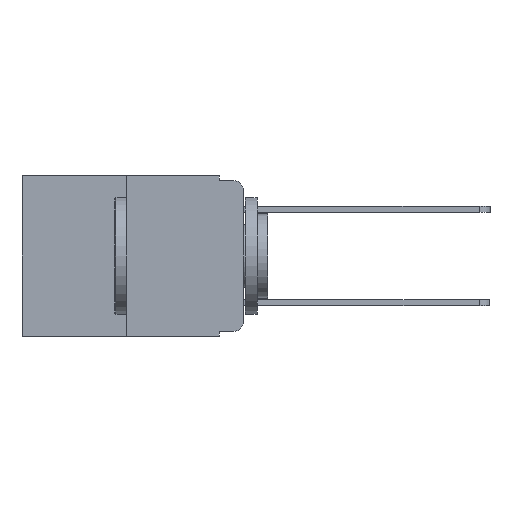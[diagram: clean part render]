
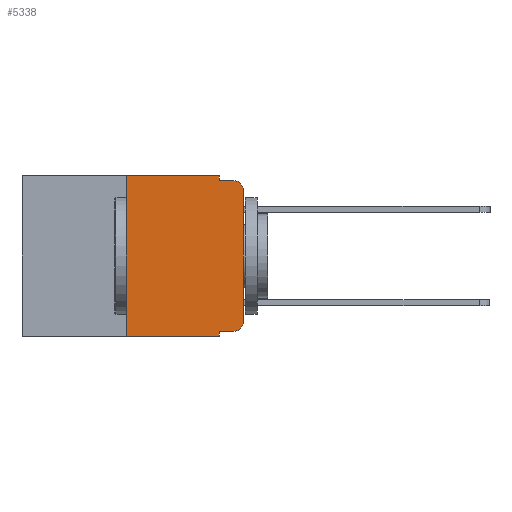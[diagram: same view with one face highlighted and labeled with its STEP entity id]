
A CAD part, left-side view. The second image highlights one B-rep face of the part: STEP entity #5338.
In plain terms, the highlighted planar face has unit normal (-1, 0, 0).
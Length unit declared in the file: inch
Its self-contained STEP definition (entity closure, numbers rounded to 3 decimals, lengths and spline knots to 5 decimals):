
#189 = CIRCLE ( 'NONE', #2507, 0.02 ) ;
#321 = EDGE_CURVE ( 'NONE', #970, #2202, #3311, .T. ) ;
#327 = ORIENTED_EDGE ( 'NONE', *, *, #11751, .T. ) ;
#368 = CARTESIAN_POINT ( 'NONE',  ( 0., 0.473, 0. ) ) ;
#484 = VERTEX_POINT ( 'NONE', #5245 ) ;
#970 = VERTEX_POINT ( 'NONE', #9499 ) ;
#1048 = EDGE_CURVE ( 'NONE', #1495, #7305, #7095, .T. ) ;
#1229 = EDGE_CURVE ( 'NONE', #1495, #2202, #2308, .T. ) ;
#1413 = CARTESIAN_POINT ( 'NONE',  ( 0., 0.02, -0.03 ) ) ;
#1495 = VERTEX_POINT ( 'NONE', #3826 ) ;
#1703 = AXIS2_PLACEMENT_3D ( 'NONE', #368, #11170, #5492 ) ;
#1918 = CARTESIAN_POINT ( 'NONE',  ( 0., 0.051, -0.01 ) ) ;
#1962 = VERTEX_POINT ( 'NONE', #1918 ) ;
#2202 = VERTEX_POINT ( 'NONE', #9196 ) ;
#2308 = LINE ( 'NONE', #10775, #7242 ) ;
#2401 = CARTESIAN_POINT ( 'NONE',  ( 0., 0.02, -0.01 ) ) ;
#2425 = FACE_OUTER_BOUND ( 'NONE', #11619, .T. ) ;
#2480 = EDGE_CURVE ( 'NONE', #5399, #1962, #8174, .T. ) ;
#2504 = DIRECTION ( 'NONE',  ( 0., 0., -1. ) ) ;
#2507 = AXIS2_PLACEMENT_3D ( 'NONE', #4015, #10698, #4992 ) ;
#2570 = PLANE ( 'NONE',  #1703 ) ;
#2672 = CARTESIAN_POINT ( 'NONE',  ( 0., 0., 0. ) ) ;
#3140 = VECTOR ( 'NONE', #8486, 39.37008 ) ;
#3311 = LINE ( 'NONE', #6581, #3622 ) ;
#3426 = CARTESIAN_POINT ( 'NONE',  ( 0., 0.051, 0. ) ) ;
#3622 = VECTOR ( 'NONE', #11095, 39.37008 ) ;
#3826 = CARTESIAN_POINT ( 'NONE',  ( 0., 0.25, -0.343 ) ) ;
#4003 = DIRECTION ( 'NONE',  ( 0., -1., 0. ) ) ;
#4015 = CARTESIAN_POINT ( 'NONE',  ( 0., 0.02, -0.313 ) ) ;
#4324 = DIRECTION ( 'NONE',  ( 0., -1., 0. ) ) ;
#4512 = EDGE_CURVE ( 'NONE', #1962, #9073, #8993, .T. ) ;
#4585 = ORIENTED_EDGE ( 'NONE', *, *, #6450, .T. ) ;
#4618 = CARTESIAN_POINT ( 'NONE',  ( 0., 0.25, 0. ) ) ;
#4736 = ORIENTED_EDGE ( 'NONE', *, *, #2480, .F. ) ;
#4833 = VECTOR ( 'NONE', #10404, 39.37008 ) ;
#4847 = DIRECTION ( 'NONE',  ( 0., -1., 0. ) ) ;
#4992 = DIRECTION ( 'NONE',  ( 0., 0., -1. ) ) ;
#5245 = CARTESIAN_POINT ( 'NONE',  ( 0., 0.02, -0.333 ) ) ;
#5319 = CIRCLE ( 'NONE', #10124, 0.02 ) ;
#5338 = ADVANCED_FACE ( 'NONE', ( #2425 ), #2570, .F. ) ;
#5399 = VERTEX_POINT ( 'NONE', #3426 ) ;
#5492 = DIRECTION ( 'NONE',  ( 0., 0., -1. ) ) ;
#5630 = VECTOR ( 'NONE', #7094, 39.37008 ) ;
#5748 = LINE ( 'NONE', #2672, #3140 ) ;
#6153 = VERTEX_POINT ( 'NONE', #9688 ) ;
#6192 = VERTEX_POINT ( 'NONE', #9721 ) ;
#6384 = ORIENTED_EDGE ( 'NONE', *, *, #7096, .T. ) ;
#6450 = EDGE_CURVE ( 'NONE', #6192, #9073, #5319, .T. ) ;
#6581 = CARTESIAN_POINT ( 'NONE',  ( 0., 0.051, 0. ) ) ;
#6741 = CARTESIAN_POINT ( 'NONE',  ( 0., 0.051, -0.333 ) ) ;
#6828 = ORIENTED_EDGE ( 'NONE', *, *, #10478, .T. ) ;
#7094 = DIRECTION ( 'NONE',  ( 0., 0., -1. ) ) ;
#7095 = LINE ( 'NONE', #4618, #4833 ) ;
#7096 = EDGE_CURVE ( 'NONE', #6153, #6192, #5748, .T. ) ;
#7199 = CARTESIAN_POINT ( 'NONE',  ( 0., 0.051, 0. ) ) ;
#7242 = VECTOR ( 'NONE', #4324, 39.37008 ) ;
#7305 = VERTEX_POINT ( 'NONE', #8837 ) ;
#7765 = VECTOR ( 'NONE', #4003, 39.37008 ) ;
#7874 = DIRECTION ( 'NONE',  ( 0., -1., 0. ) ) ;
#8072 = LINE ( 'NONE', #10683, #7765 ) ;
#8174 = LINE ( 'NONE', #7199, #5630 ) ;
#8181 = ORIENTED_EDGE ( 'NONE', *, *, #1229, .T. ) ;
#8301 = ORIENTED_EDGE ( 'NONE', *, *, #321, .F. ) ;
#8334 = DIRECTION ( 'NONE',  ( -1., 0., 0. ) ) ;
#8471 = ORIENTED_EDGE ( 'NONE', *, *, #9312, .F. ) ;
#8486 = DIRECTION ( 'NONE',  ( 0., 0., 1. ) ) ;
#8681 = VECTOR ( 'NONE', #7874, 39.37008 ) ;
#8837 = CARTESIAN_POINT ( 'NONE',  ( 0., 0.25, 0. ) ) ;
#8993 = LINE ( 'NONE', #10678, #8681 ) ;
#9073 = VERTEX_POINT ( 'NONE', #2401 ) ;
#9196 = CARTESIAN_POINT ( 'NONE',  ( 0., 0.051, -0.343 ) ) ;
#9312 = EDGE_CURVE ( 'NONE', #7305, #5399, #8072, .T. ) ;
#9351 = ORIENTED_EDGE ( 'NONE', *, *, #1048, .F. ) ;
#9496 = LINE ( 'NONE', #6741, #11720 ) ;
#9499 = CARTESIAN_POINT ( 'NONE',  ( 0., 0.051, -0.333 ) ) ;
#9688 = CARTESIAN_POINT ( 'NONE',  ( 0., 0., -0.313 ) ) ;
#9721 = CARTESIAN_POINT ( 'NONE',  ( 0., 0., -0.03 ) ) ;
#10124 = AXIS2_PLACEMENT_3D ( 'NONE', #1413, #8334, #2504 ) ;
#10404 = DIRECTION ( 'NONE',  ( 0., 0., 1. ) ) ;
#10478 = EDGE_CURVE ( 'NONE', #484, #6153, #189, .T. ) ;
#10678 = CARTESIAN_POINT ( 'NONE',  ( 0., 0.051, -0.01 ) ) ;
#10683 = CARTESIAN_POINT ( 'NONE',  ( 0., 0.473, 0. ) ) ;
#10698 = DIRECTION ( 'NONE',  ( -1., 0., 0. ) ) ;
#10765 = ORIENTED_EDGE ( 'NONE', *, *, #4512, .F. ) ;
#10775 = CARTESIAN_POINT ( 'NONE',  ( 0., 0.473, -0.343 ) ) ;
#11095 = DIRECTION ( 'NONE',  ( 0., 0., -1. ) ) ;
#11170 = DIRECTION ( 'NONE',  ( 1., 0., 0. ) ) ;
#11619 = EDGE_LOOP ( 'NONE', ( #6384, #4585, #10765, #4736, #8471, #9351, #8181, #8301, #327, #6828 ) ) ;
#11720 = VECTOR ( 'NONE', #4847, 39.37008 ) ;
#11751 = EDGE_CURVE ( 'NONE', #970, #484, #9496, .T. ) ;
